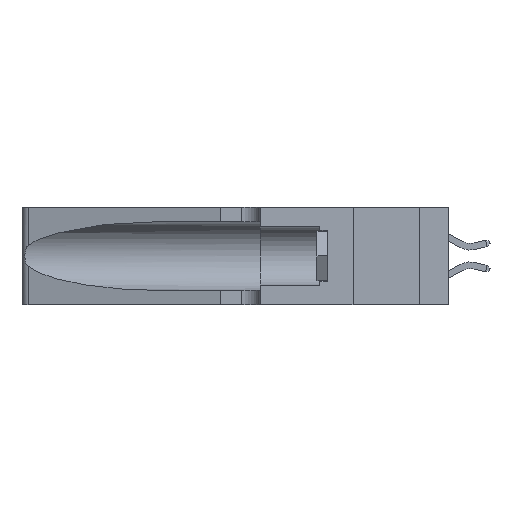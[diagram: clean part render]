
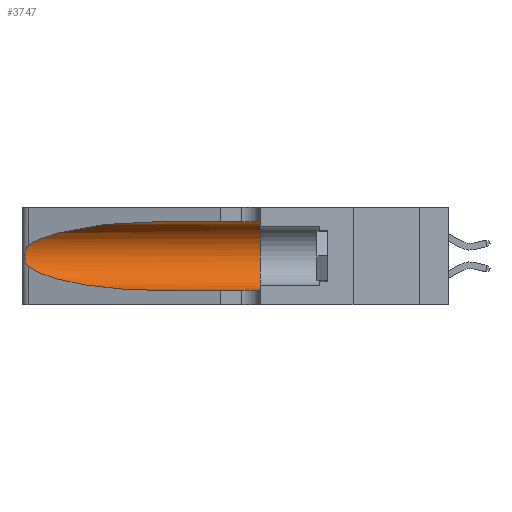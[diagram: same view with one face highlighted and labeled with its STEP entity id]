
A CAD part, left-side view. The second image highlights one B-rep face of the part: STEP entity #3747.
In plain terms, the highlighted cylindrical face has radius 3.308 mm (diameter 6.617 mm), a partial arc.
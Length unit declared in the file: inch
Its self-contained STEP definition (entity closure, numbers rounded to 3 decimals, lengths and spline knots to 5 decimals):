
#268 = CARTESIAN_POINT ( 'NONE',  ( 0.25639, 1.23186, 0.15144 ) ) ;
#342 = CARTESIAN_POINT ( 'NONE',  ( 0.25856, 1.23593, 0.16098 ) ) ;
#805 = AXIS2_PLACEMENT_3D ( 'NONE', #18517, #15868, #14295 ) ;
#808 = CIRCLE ( 'NONE', #17393, 0.13025 ) ;
#1373 = EDGE_CURVE ( 'NONE', #1429, #4803, #18400, .T. ) ;
#1377 = B_SPLINE_CURVE_WITH_KNOTS ( 'NONE', 3,
 ( #16084, #11768, #7582, #8827, #3288, #10440, #17628, #7465, #6097, #342, #16141, #268, #4481, #1833 ),
 .UNSPECIFIED., .F., .F.,
 ( 4, 2, 2, 2, 2, 2, 4 ),
 ( 0., 0.00027, 0.00053, 0.00107, 0.0016, 0.00187, 0.00214 ),
 .UNSPECIFIED. ) ;
#1429 = VERTEX_POINT ( 'NONE', #3665 ) ;
#1447 = ORIENTED_EDGE ( 'NONE', *, *, #11693, .T. ) ;
#1515 = DIRECTION ( 'NONE',  ( 0., -1., 0. ) ) ;
#1833 = CARTESIAN_POINT ( 'NONE',  ( 0.25487, 1.22718, 0.14631 ) ) ;
#1886 = ORIENTED_EDGE ( 'NONE', *, *, #5712, .T. ) ;
#1895 = VERTEX_POINT ( 'NONE', #2958 ) ;
#2033 = ORIENTED_EDGE ( 'NONE', *, *, #1373, .T. ) ;
#2737 = DIRECTION ( 'NONE',  ( 0., -1., 0. ) ) ;
#2958 = CARTESIAN_POINT ( 'NONE',  ( 0.1305, 0.35, 0.05475 ) ) ;
#3288 = CARTESIAN_POINT ( 'NONE',  ( 0.25854, 1.2359, 0.20912 ) ) ;
#3538 = EDGE_CURVE ( 'NONE', #8237, #1895, #808, .T. ) ;
#3665 = CARTESIAN_POINT ( 'NONE',  ( 0.25487, 1.22718, 0.14631 ) ) ;
#3747 = ADVANCED_FACE ( 'NONE', ( #8820 ), #13102, .F. ) ;
#3772 = DIRECTION ( 'NONE',  ( 0., 1., 0. ) ) ;
#4481 = CARTESIAN_POINT ( 'NONE',  ( 0.25555, 1.22993, 0.14849 ) ) ;
#4574 = ORIENTED_EDGE ( 'NONE', *, *, #11557, .F. ) ;
#4803 = VERTEX_POINT ( 'NONE', #11101 ) ;
#5712 = EDGE_CURVE ( 'NONE', #8607, #16768, #12497, .T. ) ;
#5851 = CARTESIAN_POINT ( 'NONE',  ( 0.18966, 0.96281, 0.05475 ) ) ;
#6097 = CARTESIAN_POINT ( 'NONE',  ( 0.26017, 1.23833, 0.17102 ) ) ;
#7465 = CARTESIAN_POINT ( 'NONE',  ( 0.26075, 1.23896, 0.178 ) ) ;
#7582 = CARTESIAN_POINT ( 'NONE',  ( 0.25639, 1.23184, 0.21858 ) ) ;
#8237 = VERTEX_POINT ( 'NONE', #14425 ) ;
#8607 = VERTEX_POINT ( 'NONE', #16710 ) ;
#8820 = FACE_OUTER_BOUND ( 'NONE', #16460, .T. ) ;
#8827 = CARTESIAN_POINT ( 'NONE',  ( 0.25787, 1.23484, 0.2124 ) ) ;
#9123 = VECTOR ( 'NONE', #1515, 39.37008 ) ;
#9172 = CARTESIAN_POINT ( 'NONE',  ( 0.1305, 0.72297, 0.31525 ) ) ;
#9607 = CARTESIAN_POINT ( 'NONE',  ( 0.1305, 0.35, 0.185 ) ) ;
#10120 = CARTESIAN_POINT ( 'NONE',  ( 0.25487, 1.22718, 0.14631 ) ) ;
#10359 = ORIENTED_EDGE ( 'NONE', *, *, #15122, .T. ) ;
#10420 = ORIENTED_EDGE ( 'NONE', *, *, #3538, .F. ) ;
#10440 = CARTESIAN_POINT ( 'NONE',  ( 0.26018, 1.23835, 0.19895 ) ) ;
#10616 = CARTESIAN_POINT ( 'NONE',  ( 0.2373, 1.15595, 0.28018 ) ) ;
#10920 = CARTESIAN_POINT ( 'NONE',  ( 0.1305, 1.61858, 0.05475 ) ) ;
#11101 = CARTESIAN_POINT ( 'NONE',  ( 0.1305, 0.72297, 0.05475 ) ) ;
#11557 = EDGE_CURVE ( 'NONE', #8607, #8237, #15899, .T. ) ;
#11693 = EDGE_CURVE ( 'NONE', #4803, #1895, #13403, .T. ) ;
#11768 = CARTESIAN_POINT ( 'NONE',  ( 0.25555, 1.22994, 0.2215 ) ) ;
#11875 = CARTESIAN_POINT ( 'NONE',  ( 0.18966, 0.96281, 0.31525 ) ) ;
#12497 =( BOUNDED_CURVE ( )  B_SPLINE_CURVE ( 3, ( #9172, #11875, #10616, #14718 ),
 .UNSPECIFIED., .F., .T. ) 
 B_SPLINE_CURVE_WITH_KNOTS ( ( 4, 4 ),
 ( 1.5708, 2.84003 ),
 .UNSPECIFIED. ) 
 CURVE ( )  GEOMETRIC_REPRESENTATION_ITEM ( )  RATIONAL_B_SPLINE_CURVE ( ( 1., 0.87, 0.87, 1. ) ) 
 REPRESENTATION_ITEM ( '' )  );
#13102 = CYLINDRICAL_SURFACE ( 'NONE', #805, 0.13025 ) ;
#13175 = VECTOR ( 'NONE', #2737, 39.37008 ) ;
#13403 = LINE ( 'NONE', #10920, #9123 ) ;
#14295 = DIRECTION ( 'NONE',  ( 0., 0., -1. ) ) ;
#14420 = CARTESIAN_POINT ( 'NONE',  ( 0.2373, 1.15595, 0.08982 ) ) ;
#14425 = CARTESIAN_POINT ( 'NONE',  ( 0.1305, 0.35, 0.31525 ) ) ;
#14718 = CARTESIAN_POINT ( 'NONE',  ( 0.25487, 1.22718, 0.22369 ) ) ;
#15122 = EDGE_CURVE ( 'NONE', #16768, #1429, #1377, .T. ) ;
#15150 = DIRECTION ( 'NONE',  ( 0., 0., 1. ) ) ;
#15672 = CARTESIAN_POINT ( 'NONE',  ( 0.1305, 1.61858, 0.31525 ) ) ;
#15714 = CARTESIAN_POINT ( 'NONE',  ( 0.25487, 1.22718, 0.22369 ) ) ;
#15868 = DIRECTION ( 'NONE',  ( 0., -1., 0. ) ) ;
#15899 = LINE ( 'NONE', #15672, #13175 ) ;
#16084 = CARTESIAN_POINT ( 'NONE',  ( 0.25487, 1.22718, 0.22369 ) ) ;
#16141 = CARTESIAN_POINT ( 'NONE',  ( 0.25789, 1.23486, 0.15765 ) ) ;
#16460 = EDGE_LOOP ( 'NONE', ( #1886, #10359, #2033, #1447, #10420, #4574 ) ) ;
#16710 = CARTESIAN_POINT ( 'NONE',  ( 0.1305, 0.72297, 0.31525 ) ) ;
#16768 = VERTEX_POINT ( 'NONE', #15714 ) ;
#17319 = CARTESIAN_POINT ( 'NONE',  ( 0.1305, 0.72297, 0.05475 ) ) ;
#17393 = AXIS2_PLACEMENT_3D ( 'NONE', #9607, #3772, #15150 ) ;
#17628 = CARTESIAN_POINT ( 'NONE',  ( 0.26075, 1.23896, 0.19203 ) ) ;
#18400 =( BOUNDED_CURVE ( )  B_SPLINE_CURVE ( 3, ( #10120, #14420, #5851, #17319 ),
 .UNSPECIFIED., .F., .T. ) 
 B_SPLINE_CURVE_WITH_KNOTS ( ( 4, 4 ),
 ( 3.44316, 4.71239 ),
 .UNSPECIFIED. ) 
 CURVE ( )  GEOMETRIC_REPRESENTATION_ITEM ( )  RATIONAL_B_SPLINE_CURVE ( ( 1., 0.87, 0.87, 1. ) ) 
 REPRESENTATION_ITEM ( '' )  );
#18517 = CARTESIAN_POINT ( 'NONE',  ( 0.1305, 1.61858, 0.185 ) ) ;
